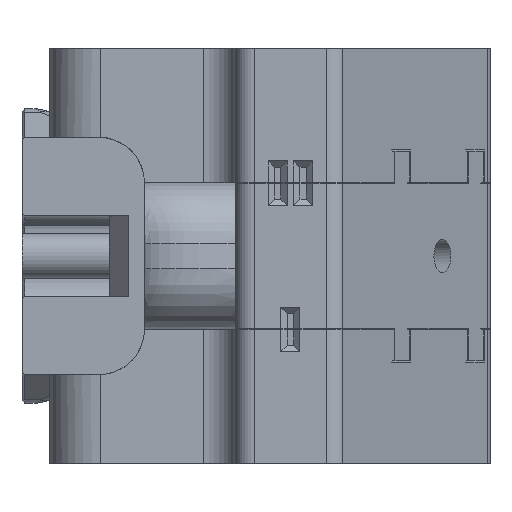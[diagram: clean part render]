
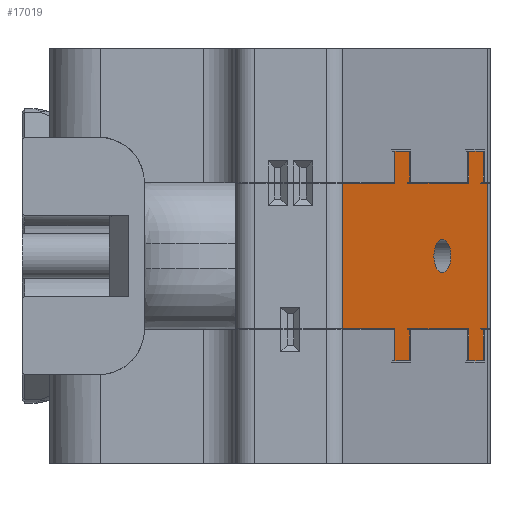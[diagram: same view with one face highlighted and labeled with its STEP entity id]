
A CAD part, left-side view. The second image highlights one B-rep face of the part: STEP entity #17019.
In plain terms, the highlighted planar face has unit normal (-0.5, -0.866, 0).
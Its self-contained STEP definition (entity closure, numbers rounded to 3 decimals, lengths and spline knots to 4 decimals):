
#1632=FACE_BOUND($,#3419,.T.);
#1818=CIRCLE($,#18096,0.2653);
#2353=FACE_OUTER_BOUND($,#3418,.T.);
#3418=EDGE_LOOP($,(#11493,#11494,#11495,#11496,#11497,#11498,#11499,#11500,
#11501,#11502,#11503,#11504,#11505,#11506,#11507,#11508,#11509,#11510,#11511,
#11512));
#3419=EDGE_LOOP($,(#11513));
#4689=LINE($,#23271,#5902);
#4692=LINE($,#23282,#5905);
#4696=LINE($,#23291,#5909);
#4700=LINE($,#23300,#5913);
#4701=LINE($,#23302,#5914);
#4702=LINE($,#23303,#5915);
#4703=LINE($,#23305,#5916);
#4704=LINE($,#23307,#5917);
#4705=LINE($,#23309,#5918);
#4706=LINE($,#23311,#5919);
#4707=LINE($,#23313,#5920);
#4708=LINE($,#23314,#5921);
#4709=LINE($,#23316,#5922);
#4710=LINE($,#23318,#5923);
#4711=LINE($,#23320,#5924);
#4712=LINE($,#23322,#5925);
#4713=LINE($,#23324,#5926);
#4714=LINE($,#23325,#5927);
#4715=LINE($,#23327,#5928);
#4716=LINE($,#23328,#5929);
#5902=VECTOR($,#19446,1.6318);
#5905=VECTOR($,#19455,0.5);
#5909=VECTOR($,#19461,0.5);
#5913=VECTOR($,#19467,0.1267);
#5914=VECTOR($,#19468,2.2819);
#5915=VECTOR($,#19469,0.1267);
#5916=VECTOR($,#19470,0.4619);
#5917=VECTOR($,#19471,0.5);
#5918=VECTOR($,#19472,1.8475);
#5919=VECTOR($,#19473,0.5);
#5920=VECTOR($,#19474,0.4619);
#5921=VECTOR($,#19475,0.5);
#5922=VECTOR($,#19476,2.2819);
#5923=VECTOR($,#19477,1.6318);
#5924=VECTOR($,#19478,0.5);
#5925=VECTOR($,#19479,0.4619);
#5926=VECTOR($,#19480,0.5);
#5927=VECTOR($,#19481,1.8475);
#5928=VECTOR($,#19482,0.4619);
#5929=VECTOR($,#19483,0.5);
#7103=VERTEX_POINT($,#23268);
#7104=VERTEX_POINT($,#23270);
#7108=VERTEX_POINT($,#23280);
#7109=VERTEX_POINT($,#23281);
#7112=VERTEX_POINT($,#23289);
#7113=VERTEX_POINT($,#23290);
#7116=VERTEX_POINT($,#23298);
#7117=VERTEX_POINT($,#23299);
#7118=VERTEX_POINT($,#23301);
#7119=VERTEX_POINT($,#23304);
#7120=VERTEX_POINT($,#23306);
#7121=VERTEX_POINT($,#23308);
#7122=VERTEX_POINT($,#23310);
#7123=VERTEX_POINT($,#23312);
#7124=VERTEX_POINT($,#23315);
#7125=VERTEX_POINT($,#23317);
#7126=VERTEX_POINT($,#23319);
#7127=VERTEX_POINT($,#23321);
#7128=VERTEX_POINT($,#23323);
#7129=VERTEX_POINT($,#23326);
#7130=VERTEX_POINT($,#23329);
#8820=EDGE_CURVE($,#7104,#7103,#4689,.T.);
#8825=EDGE_CURVE($,#7108,#7109,#4692,.F.);
#8829=EDGE_CURVE($,#7112,#7113,#4696,.F.);
#8833=EDGE_CURVE($,#7116,#7117,#4700,.T.);
#8834=EDGE_CURVE($,#7118,#7117,#4701,.T.);
#8835=EDGE_CURVE($,#7118,#7109,#4702,.T.);
#8836=EDGE_CURVE($,#7119,#7108,#4703,.F.);
#8837=EDGE_CURVE($,#7120,#7119,#4704,.F.);
#8838=EDGE_CURVE($,#7120,#7121,#4705,.T.);
#8839=EDGE_CURVE($,#7122,#7121,#4706,.F.);
#8840=EDGE_CURVE($,#7123,#7122,#4707,.F.);
#8841=EDGE_CURVE($,#7104,#7123,#4708,.F.);
#8842=EDGE_CURVE($,#7124,#7103,#4709,.T.);
#8843=EDGE_CURVE($,#7124,#7125,#4710,.T.);
#8844=EDGE_CURVE($,#7126,#7125,#4711,.F.);
#8845=EDGE_CURVE($,#7127,#7126,#4712,.T.);
#8846=EDGE_CURVE($,#7128,#7127,#4713,.F.);
#8847=EDGE_CURVE($,#7128,#7113,#4714,.T.);
#8848=EDGE_CURVE($,#7129,#7112,#4715,.T.);
#8849=EDGE_CURVE($,#7116,#7129,#4716,.F.);
#8850=EDGE_CURVE($,#7130,#7130,#1818,.T.);
#11493=ORIENTED_EDGE($,*,*,#8833,.T.);
#11494=ORIENTED_EDGE($,*,*,#8834,.F.);
#11495=ORIENTED_EDGE($,*,*,#8835,.T.);
#11496=ORIENTED_EDGE($,*,*,#8825,.F.);
#11497=ORIENTED_EDGE($,*,*,#8836,.F.);
#11498=ORIENTED_EDGE($,*,*,#8837,.F.);
#11499=ORIENTED_EDGE($,*,*,#8838,.T.);
#11500=ORIENTED_EDGE($,*,*,#8839,.F.);
#11501=ORIENTED_EDGE($,*,*,#8840,.F.);
#11502=ORIENTED_EDGE($,*,*,#8841,.F.);
#11503=ORIENTED_EDGE($,*,*,#8820,.T.);
#11504=ORIENTED_EDGE($,*,*,#8842,.F.);
#11505=ORIENTED_EDGE($,*,*,#8843,.T.);
#11506=ORIENTED_EDGE($,*,*,#8844,.F.);
#11507=ORIENTED_EDGE($,*,*,#8845,.F.);
#11508=ORIENTED_EDGE($,*,*,#8846,.F.);
#11509=ORIENTED_EDGE($,*,*,#8847,.T.);
#11510=ORIENTED_EDGE($,*,*,#8829,.F.);
#11511=ORIENTED_EDGE($,*,*,#8848,.F.);
#11512=ORIENTED_EDGE($,*,*,#8849,.F.);
#11513=ORIENTED_EDGE($,*,*,#8850,.T.);
#16678=PLANE($,#18095);
#17019=ADVANCED_FACE($,(#2353,#1632),#16678,.F.);
#18095=AXIS2_PLACEMENT_3D($,#23297,#19465,#19466);
#18096=AXIS2_PLACEMENT_3D($,#23330,#19484,#19485);
#19446=DIRECTION($,(-0.866,0.5,0.));
#19455=DIRECTION($,(0.,0.,1.));
#19461=DIRECTION($,(0.,0.,-1.));
#19465=DIRECTION('center_axis',(0.5,0.866,0.));
#19466=DIRECTION('ref_axis',(-0.75,0.433,-0.5));
#19467=DIRECTION($,(0.866,-0.5,0.));
#19468=DIRECTION($,(0.,0.,-1.));
#19469=DIRECTION($,(-0.866,0.5,0.));
#19470=DIRECTION($,(-0.866,0.5,0.));
#19471=DIRECTION($,(0.,0.,-1.));
#19472=DIRECTION($,(-0.866,0.5,0.));
#19473=DIRECTION($,(0.,0.,1.));
#19474=DIRECTION($,(-0.866,0.5,0.));
#19475=DIRECTION($,(0.,0.,-1.));
#19476=DIRECTION($,(0.,0.,1.));
#19477=DIRECTION($,(0.866,-0.5,0.));
#19478=DIRECTION($,(0.,0.,-1.));
#19479=DIRECTION($,(-0.866,0.5,0.));
#19480=DIRECTION($,(0.,0.,1.));
#19481=DIRECTION($,(0.866,-0.5,0.));
#19482=DIRECTION($,(-0.866,0.5,0.));
#19483=DIRECTION($,(0.,0.,1.));
#19484=DIRECTION('center_axis',(0.5,0.866,0.));
#19485=DIRECTION('ref_axis',(0.866,-0.5,0.));
#23268=CARTESIAN_POINT('',(-18.3416,-4.4441,1.2409));
#23270=CARTESIAN_POINT('',(-16.9284,-5.26,1.2409));
#23271=CARTESIAN_POINT($,(-14.6292,-6.5875,1.2409));
#23280=CARTESIAN_POINT('',(-14.5284,-6.6457,1.7409));
#23281=CARTESIAN_POINT('',(-14.5284,-6.6457,1.2409));
#23282=CARTESIAN_POINT($,(-14.5284,-6.6457,0.8955));
#23289=CARTESIAN_POINT('',(-14.9284,-6.4147,-1.5409));
#23290=CARTESIAN_POINT('',(-14.9284,-6.4147,-1.0409));
#23291=CARTESIAN_POINT($,(-14.9284,-6.4147,0.8955));
#23297=CARTESIAN_POINT('Origin',(-15.9303,-5.8363,0.446));
#23298=CARTESIAN_POINT('',(-14.5284,-6.6457,-1.0409));
#23299=CARTESIAN_POINT('',(-14.4187,-6.709,-1.0409));
#23300=CARTESIAN_POINT($,(-14.6292,-6.5875,-1.0409));
#23301=CARTESIAN_POINT('',(-14.4187,-6.709,1.2409));
#23302=CARTESIAN_POINT($,(-14.4187,-6.709,2.123));
#23303=CARTESIAN_POINT($,(-14.6292,-6.5875,1.2409));
#23304=CARTESIAN_POINT('',(-14.9284,-6.4147,1.7409));
#23305=CARTESIAN_POINT($,(-15.2124,-6.2508,1.7409));
#23306=CARTESIAN_POINT('',(-14.9284,-6.4147,1.2409));
#23307=CARTESIAN_POINT($,(-14.9284,-6.4147,0.8955));
#23308=CARTESIAN_POINT('',(-16.5284,-5.491,1.2409));
#23309=CARTESIAN_POINT($,(-14.6292,-6.5875,1.2409));
#23310=CARTESIAN_POINT('',(-16.5284,-5.491,1.7409));
#23311=CARTESIAN_POINT($,(-16.5284,-5.491,1.3435));
#23312=CARTESIAN_POINT('',(-16.9284,-5.26,1.7409));
#23313=CARTESIAN_POINT($,(-16.5443,-5.4818,1.7409));
#23314=CARTESIAN_POINT($,(-16.9284,-5.26,1.3435));
#23315=CARTESIAN_POINT('',(-18.3416,-4.4441,-1.0409));
#23316=CARTESIAN_POINT($,(-18.3416,-4.4441,0.273));
#23317=CARTESIAN_POINT('',(-16.9284,-5.26,-1.0409));
#23318=CARTESIAN_POINT($,(-14.6292,-6.5875,-1.0409));
#23319=CARTESIAN_POINT('',(-16.9284,-5.26,-1.5409));
#23320=CARTESIAN_POINT($,(-16.9284,-5.26,-0.7974));
#23321=CARTESIAN_POINT('',(-16.5284,-5.491,-1.5409));
#23322=CARTESIAN_POINT($,(-16.5443,-5.4818,-1.5409));
#23323=CARTESIAN_POINT('',(-16.5284,-5.491,-1.0409));
#23324=CARTESIAN_POINT($,(-16.5284,-5.491,-0.7974));
#23325=CARTESIAN_POINT($,(-14.6292,-6.5875,-1.0409));
#23326=CARTESIAN_POINT('',(-14.5284,-6.6457,-1.5409));
#23327=CARTESIAN_POINT($,(-15.2124,-6.2508,-1.5409));
#23328=CARTESIAN_POINT($,(-14.5284,-6.6457,0.8955));
#23329=CARTESIAN_POINT('',(-15.8707,-5.8707,0.1));
#23330=CARTESIAN_POINT('Origin',(-15.641,-6.0033,0.1));
